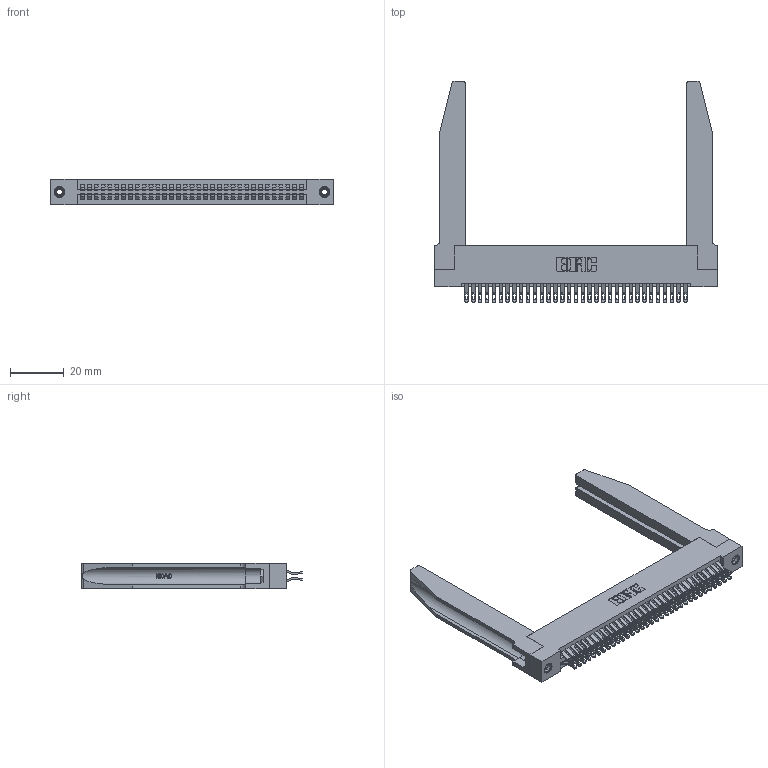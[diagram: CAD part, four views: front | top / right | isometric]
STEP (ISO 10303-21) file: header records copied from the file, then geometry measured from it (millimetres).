
FILE_DESCRIPTION (( 'STEP AP203' ), '1' );
FILE_NAME ('395-066-555-278.STEP', '2019-10-23T21:07:57', ( '' ), ( '' ), 'SwSTEP 2.0', 'SolidWorks 2016', '' );
FILE_SCHEMA (( 'CONFIG_CONTROL_DESIGN' ));
Length unit declared in the file: inch
Products named in the file (5): 345-292-001_555 Tail; 345-250-001_345-250-001-102; 345-220-078_345-220-078; 395-066-555-278; 345 Part_Flush Mounting Lugs - 0.156 Dia-TH
Assembly tree (71 placements, depth 2):
  395-066-555-278
    345 Part_Flush Mounting Lugs - 0.156 Dia-TH
    345-292-001_555 Tail  x66
    345-250-001_345-250-001-102  x2
    345-220-078_345-220-078  x2
Bounding box: 105.05 x 82.09 x 9.4 mm (x, y, z)
Volume: 18083.4 mm3; surface area: 22574.3 mm2
Topology: 71 solids, 71 shells, 4056 faces, 12631 edges, 8410 vertices
Faces by surface type: plane 2268, cylinder 1736, bspline 36, cone 12, torus 4
Entity records: 32170 total; most frequent: CARTESIAN_POINT 6353, ORIENTED_EDGE 5154, DIRECTION 4575, EDGE_CURVE 2577, LINE 2199, VECTOR 2199, VERTEX_POINT 1712, AXIS2_PLACEMENT_3D 1188
